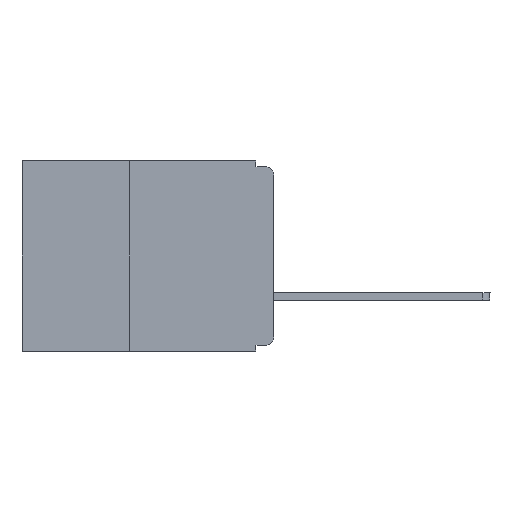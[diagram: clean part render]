
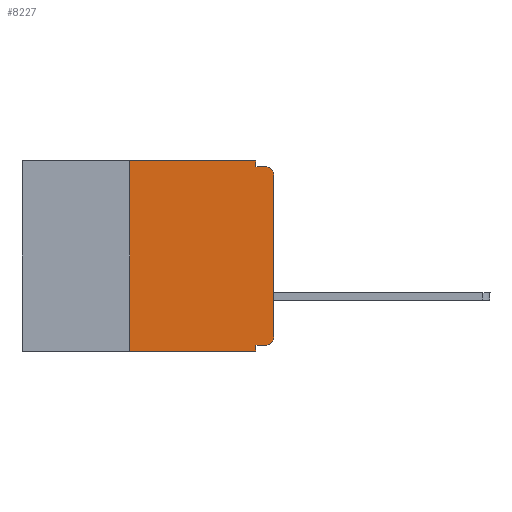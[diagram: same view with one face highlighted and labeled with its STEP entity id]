
A CAD part, left-side view. The second image highlights one B-rep face of the part: STEP entity #8227.
In plain terms, the highlighted planar face has unit normal (-1, 0, 0).
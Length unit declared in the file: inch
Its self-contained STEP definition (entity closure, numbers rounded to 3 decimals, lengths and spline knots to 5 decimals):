
#381 = CARTESIAN_POINT ( 'NONE',  ( 0., 0.437, -0.33 ) ) ;
#501 = EDGE_LOOP ( 'NONE', ( #600, #8884, #3733, #5799, #4495, #11495, #1931, #5035, #6258, #12303 ) ) ;
#600 = ORIENTED_EDGE ( 'NONE', *, *, #2808, .T. ) ;
#737 = CARTESIAN_POINT ( 'NONE',  ( 0., 0.015, -0.305 ) ) ;
#808 = VERTEX_POINT ( 'NONE', #1753 ) ;
#1413 = DIRECTION ( 'NONE',  ( 0., 0., -1. ) ) ;
#1753 = CARTESIAN_POINT ( 'NONE',  ( 0., 0.25, 0. ) ) ;
#1931 = ORIENTED_EDGE ( 'NONE', *, *, #10807, .T. ) ;
#2276 = CARTESIAN_POINT ( 'NONE',  ( 0., 0.437, 0. ) ) ;
#2428 = CARTESIAN_POINT ( 'NONE',  ( 0., 0., -0.01 ) ) ;
#2517 = LINE ( 'NONE', #4433, #13373 ) ;
#2598 = LINE ( 'NONE', #3317, #13472 ) ;
#2808 = EDGE_CURVE ( 'NONE', #13339, #7343, #12496, .T. ) ;
#3062 = VECTOR ( 'NONE', #5777, 39.37008 ) ;
#3292 = CARTESIAN_POINT ( 'NONE',  ( 0., 0.015, -0.32 ) ) ;
#3304 = CIRCLE ( 'NONE', #8678, 0.015 ) ;
#3317 = CARTESIAN_POINT ( 'NONE',  ( 0., 0.031, -0.33 ) ) ;
#3384 = VERTEX_POINT ( 'NONE', #3292 ) ;
#3434 = EDGE_CURVE ( 'NONE', #6732, #6619, #10788, .T. ) ;
#3733 = ORIENTED_EDGE ( 'NONE', *, *, #3434, .F. ) ;
#3782 = VECTOR ( 'NONE', #11705, 39.37008 ) ;
#3976 = CARTESIAN_POINT ( 'NONE',  ( 0., 0.031, -0.33 ) ) ;
#4015 = DIRECTION ( 'NONE',  ( -1., 0., 0. ) ) ;
#4108 = VERTEX_POINT ( 'NONE', #9618 ) ;
#4139 = CARTESIAN_POINT ( 'NONE',  ( 0., 0.015, -0.025 ) ) ;
#4240 = VECTOR ( 'NONE', #8735, 39.37008 ) ;
#4242 = DIRECTION ( 'NONE',  ( 0., -1., 0. ) ) ;
#4426 = CARTESIAN_POINT ( 'NONE',  ( 0., 0., -0.305 ) ) ;
#4433 = CARTESIAN_POINT ( 'NONE',  ( 0., 0.437, 0. ) ) ;
#4495 = ORIENTED_EDGE ( 'NONE', *, *, #5302, .F. ) ;
#4993 = CARTESIAN_POINT ( 'NONE',  ( 0., 0.031, -0.32 ) ) ;
#5035 = ORIENTED_EDGE ( 'NONE', *, *, #9125, .F. ) ;
#5302 = EDGE_CURVE ( 'NONE', #808, #11943, #2517, .T. ) ;
#5482 = FACE_OUTER_BOUND ( 'NONE', #501, .T. ) ;
#5777 = DIRECTION ( 'NONE',  ( 0., -1., 0. ) ) ;
#5799 = ORIENTED_EDGE ( 'NONE', *, *, #9791, .F. ) ;
#6000 = DIRECTION ( 'NONE',  ( 0., 0., -1. ) ) ;
#6258 = ORIENTED_EDGE ( 'NONE', *, *, #9687, .F. ) ;
#6418 = LINE ( 'NONE', #381, #3062 ) ;
#6616 = VECTOR ( 'NONE', #1413, 39.37008 ) ;
#6619 = VERTEX_POINT ( 'NONE', #8966 ) ;
#6732 = VERTEX_POINT ( 'NONE', #12313 ) ;
#6789 = LINE ( 'NONE', #7616, #4240 ) ;
#6996 = VECTOR ( 'NONE', #10744, 39.37008 ) ;
#7343 = VERTEX_POINT ( 'NONE', #10207 ) ;
#7381 = CARTESIAN_POINT ( 'NONE',  ( 0., 0.25, -0.33 ) ) ;
#7530 = EDGE_CURVE ( 'NONE', #4108, #808, #11997, .T. ) ;
#7616 = CARTESIAN_POINT ( 'NONE',  ( 0., 0., -0.32 ) ) ;
#7956 = CARTESIAN_POINT ( 'NONE',  ( 0., 0.031, 0. ) ) ;
#8227 = ADVANCED_FACE ( 'NONE', ( #5482 ), #9997, .F. ) ;
#8328 = CARTESIAN_POINT ( 'NONE',  ( 0., 0.031, 0. ) ) ;
#8678 = AXIS2_PLACEMENT_3D ( 'NONE', #4139, #10797, #11980 ) ;
#8735 = DIRECTION ( 'NONE',  ( 0., 1., 0. ) ) ;
#8819 = EDGE_CURVE ( 'NONE', #3384, #13339, #8901, .T. ) ;
#8841 = DIRECTION ( 'NONE',  ( 0., 0., -1. ) ) ;
#8862 = DIRECTION ( 'NONE',  ( 0., -1., 0. ) ) ;
#8884 = ORIENTED_EDGE ( 'NONE', *, *, #13709, .T. ) ;
#8901 = CIRCLE ( 'NONE', #9611, 0.015 ) ;
#8966 = CARTESIAN_POINT ( 'NONE',  ( 0., 0.015, -0.01 ) ) ;
#9084 = VECTOR ( 'NONE', #8862, 39.37008 ) ;
#9125 = EDGE_CURVE ( 'NONE', #13634, #11941, #2598, .T. ) ;
#9500 = CARTESIAN_POINT ( 'NONE',  ( 0., 0., 0. ) ) ;
#9611 = AXIS2_PLACEMENT_3D ( 'NONE', #737, #4015, #6000 ) ;
#9618 = CARTESIAN_POINT ( 'NONE',  ( 0., 0.25, -0.33 ) ) ;
#9687 = EDGE_CURVE ( 'NONE', #3384, #13634, #6789, .T. ) ;
#9791 = EDGE_CURVE ( 'NONE', #11943, #6732, #11441, .T. ) ;
#9899 = DIRECTION ( 'NONE',  ( 0., 0., -1. ) ) ;
#9997 = PLANE ( 'NONE',  #11429 ) ;
#10207 = CARTESIAN_POINT ( 'NONE',  ( 0., 0., -0.025 ) ) ;
#10744 = DIRECTION ( 'NONE',  ( 0., 0., 1. ) ) ;
#10788 = LINE ( 'NONE', #2428, #9084 ) ;
#10797 = DIRECTION ( 'NONE',  ( -1., 0., 0. ) ) ;
#10807 = EDGE_CURVE ( 'NONE', #4108, #11941, #6418, .T. ) ;
#11429 = AXIS2_PLACEMENT_3D ( 'NONE', #2276, #13153, #9899 ) ;
#11441 = LINE ( 'NONE', #7956, #6616 ) ;
#11495 = ORIENTED_EDGE ( 'NONE', *, *, #7530, .F. ) ;
#11705 = DIRECTION ( 'NONE',  ( 0., 0., 1. ) ) ;
#11941 = VERTEX_POINT ( 'NONE', #3976 ) ;
#11943 = VERTEX_POINT ( 'NONE', #8328 ) ;
#11980 = DIRECTION ( 'NONE',  ( 0., 0., -1. ) ) ;
#11997 = LINE ( 'NONE', #7381, #6996 ) ;
#12303 = ORIENTED_EDGE ( 'NONE', *, *, #8819, .T. ) ;
#12313 = CARTESIAN_POINT ( 'NONE',  ( 0., 0.031, -0.01 ) ) ;
#12496 = LINE ( 'NONE', #9500, #3782 ) ;
#13153 = DIRECTION ( 'NONE',  ( 1., 0., 0. ) ) ;
#13339 = VERTEX_POINT ( 'NONE', #4426 ) ;
#13373 = VECTOR ( 'NONE', #4242, 39.37008 ) ;
#13472 = VECTOR ( 'NONE', #8841, 39.37008 ) ;
#13634 = VERTEX_POINT ( 'NONE', #4993 ) ;
#13709 = EDGE_CURVE ( 'NONE', #7343, #6619, #3304, .T. ) ;
